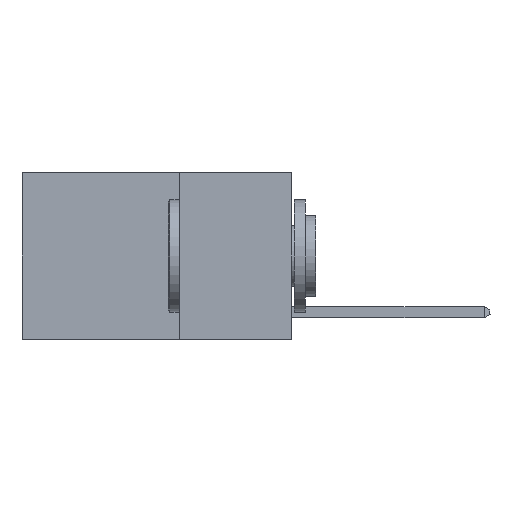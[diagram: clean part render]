
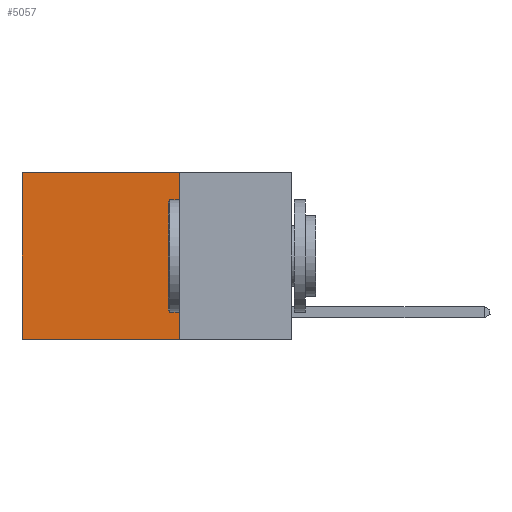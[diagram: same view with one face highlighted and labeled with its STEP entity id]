
A CAD part, left-side view. The second image highlights one B-rep face of the part: STEP entity #5057.
In plain terms, the highlighted planar face has unit normal (-1, 0, 0).
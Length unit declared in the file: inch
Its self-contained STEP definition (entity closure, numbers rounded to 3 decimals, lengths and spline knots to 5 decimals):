
#570 = DIRECTION ( 'NONE',  ( 0., 0., -1. ) ) ;
#800 = PLANE ( 'NONE',  #12319 ) ;
#885 = VECTOR ( 'NONE', #14261, 39.37008 ) ;
#1007 = ORIENTED_EDGE ( 'NONE', *, *, #9871, .T. ) ;
#1072 = VERTEX_POINT ( 'NONE', #14385 ) ;
#1864 = ORIENTED_EDGE ( 'NONE', *, *, #14287, .F. ) ;
#1953 = VERTEX_POINT ( 'NONE', #4324 ) ;
#2126 = FACE_OUTER_BOUND ( 'NONE', #4519, .T. ) ;
#3128 = DIRECTION ( 'NONE',  ( 1., 0., 0. ) ) ;
#3493 = CARTESIAN_POINT ( 'NONE',  ( 0.2625, 0.25, -0.37 ) ) ;
#3698 = EDGE_CURVE ( 'NONE', #8694, #1953, #9616, .T. ) ;
#3894 = CARTESIAN_POINT ( 'NONE',  ( 0.2625, 0.6, 0. ) ) ;
#3997 = DIRECTION ( 'NONE',  ( 0., 0., -1. ) ) ;
#4324 = CARTESIAN_POINT ( 'NONE',  ( 0.2625, 0.6, -0.37 ) ) ;
#4519 = EDGE_LOOP ( 'NONE', ( #1007, #14592, #1864, #11210 ) ) ;
#5057 = ADVANCED_FACE ( 'NONE', ( #2126 ), #800, .F. ) ;
#5479 = LINE ( 'NONE', #7423, #13378 ) ;
#7223 = CARTESIAN_POINT ( 'NONE',  ( 0.2625, 0.25, 0. ) ) ;
#7423 = CARTESIAN_POINT ( 'NONE',  ( 0.2625, 0.25, 0. ) ) ;
#8694 = VERTEX_POINT ( 'NONE', #3493 ) ;
#9616 = LINE ( 'NONE', #13154, #885 ) ;
#9861 = LINE ( 'NONE', #7223, #12449 ) ;
#9871 = EDGE_CURVE ( 'NONE', #12887, #1953, #13507, .T. ) ;
#9921 = CARTESIAN_POINT ( 'NONE',  ( 0.2625, 0.25, 0. ) ) ;
#10265 = VECTOR ( 'NONE', #570, 39.37008 ) ;
#11047 = DIRECTION ( 'NONE',  ( 0., 0., -1. ) ) ;
#11210 = ORIENTED_EDGE ( 'NONE', *, *, #11643, .T. ) ;
#11530 = CARTESIAN_POINT ( 'NONE',  ( 0.2625, 0.6, 0. ) ) ;
#11643 = EDGE_CURVE ( 'NONE', #1072, #12887, #9861, .T. ) ;
#12319 = AXIS2_PLACEMENT_3D ( 'NONE', #9921, #3128, #11047 ) ;
#12449 = VECTOR ( 'NONE', #13927, 39.37008 ) ;
#12887 = VERTEX_POINT ( 'NONE', #11530 ) ;
#13154 = CARTESIAN_POINT ( 'NONE',  ( 0.2625, 0.25, -0.37 ) ) ;
#13378 = VECTOR ( 'NONE', #3997, 39.37008 ) ;
#13507 = LINE ( 'NONE', #3894, #10265 ) ;
#13927 = DIRECTION ( 'NONE',  ( 0., 1., 0. ) ) ;
#14261 = DIRECTION ( 'NONE',  ( 0., 1., 0. ) ) ;
#14287 = EDGE_CURVE ( 'NONE', #1072, #8694, #5479, .T. ) ;
#14385 = CARTESIAN_POINT ( 'NONE',  ( 0.2625, 0.25, 0. ) ) ;
#14592 = ORIENTED_EDGE ( 'NONE', *, *, #3698, .F. ) ;
